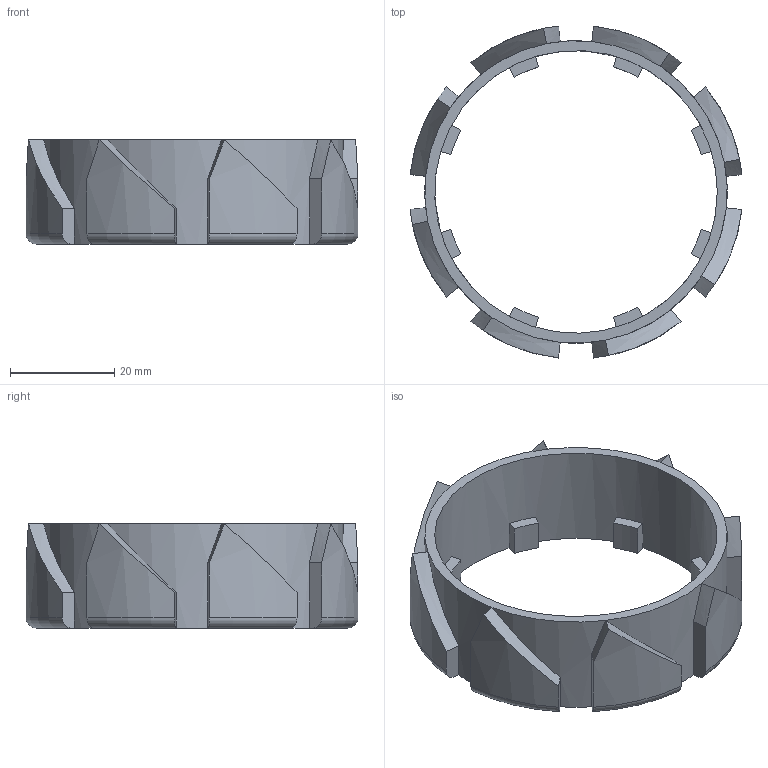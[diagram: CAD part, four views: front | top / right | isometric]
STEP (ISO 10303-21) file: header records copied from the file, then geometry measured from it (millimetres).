
FILE_DESCRIPTION((''),'2;1');
FILE_NAME('PM522INSERTRearIndexRing2.stp','2015-10-01T18:19:22',('JamesRPatrick'),(''),'Autodesk Inventor 2012','Autodesk Inventor 2012','');
FILE_SCHEMA(('AUTOMOTIVE_DESIGN { 1 0 10303 214 1 1 1 1 }'));
Length unit declared in the file: millimetre
Products named in the file (1): PM522INSERTRearIndexRing2
Bounding box: 63.65 x 63.65 x 20 mm (x, y, z)
Volume: 12924.1 mm3; surface area: 9666.5 mm2
Topology: 1 solids, 1 shells, 91 faces, 251 edges, 162 vertices
Faces by surface type: plane 42, cylinder 25, bspline 16, torus 8
Full cylindrical faces by diameter (mm): 54.2 x1
Entity records: 3154 total; most frequent: CARTESIAN_POINT 886, ORIENTED_EDGE 498, DIRECTION 434, EDGE_CURVE 249, VERTEX_POINT 161, AXIS2_PLACEMENT_3D 157, VECTOR 120, LINE 120
